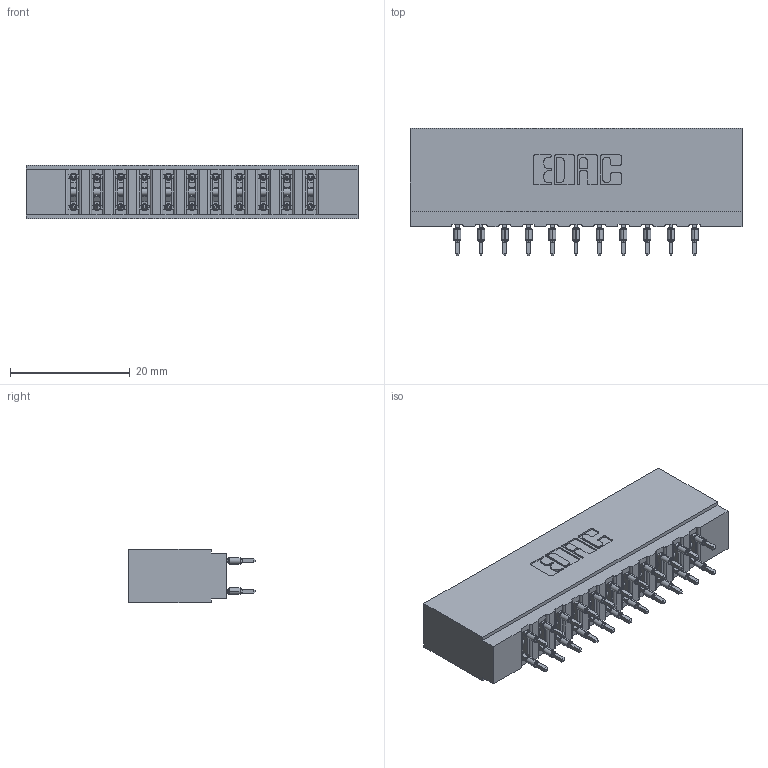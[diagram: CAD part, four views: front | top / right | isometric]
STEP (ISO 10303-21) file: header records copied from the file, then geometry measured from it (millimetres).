
FILE_DESCRIPTION (( 'STEP AP203' ), '1' );
FILE_NAME ('737-022-560-201.STEP', '2020-09-10T21:35:18', ( '' ), ( '' ), 'SwSTEP 2.0', 'SolidWorks 2020', '' );
FILE_SCHEMA (( 'CONFIG_CONTROL_DESIGN' ));
Length unit declared in the file: inch
Products named in the file (3): 737 Part_Insulator Option - 01; 745-292-001_560; 737-022-560-201
Assembly tree (23 placements, depth 2):
  737-022-560-201
    737 Part_Insulator Option - 01
    745-292-001_560  x22
Bounding box: 55.42 x 21.22 x 8.89 mm (x, y, z)
Volume: 5756.4 mm3; surface area: 8066.3 mm2
Topology: 23 solids, 23 shells, 2272 faces, 6217 edges, 3954 vertices
Faces by surface type: plane 1187, cylinder 513, bspline 440, torus 132
Entity records: 23410 total; most frequent: CARTESIAN_POINT 4577, ORIENTED_EDGE 3950, DIRECTION 3479, EDGE_CURVE 1975, VECTOR 1719, LINE 1719, VERTEX_POINT 1266, AXIS2_PLACEMENT_3D 880
